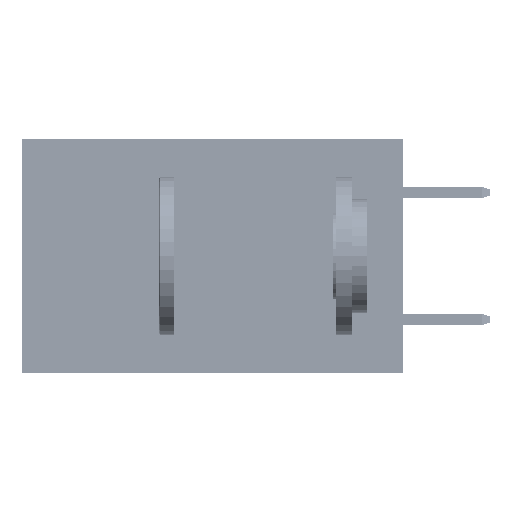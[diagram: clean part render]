
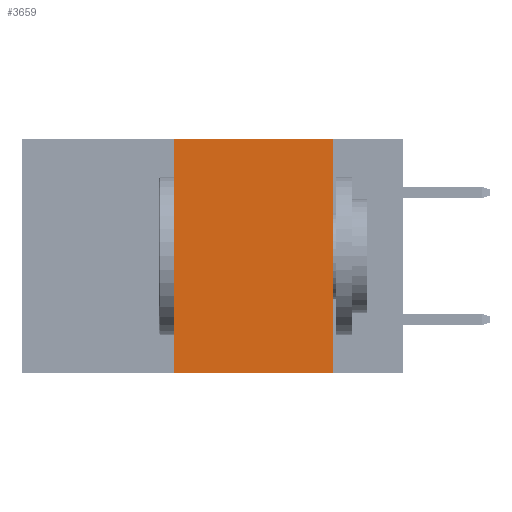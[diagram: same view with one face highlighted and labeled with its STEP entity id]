
A CAD part, left-side view. The second image highlights one B-rep face of the part: STEP entity #3659.
In plain terms, the highlighted planar face has unit normal (-1, 0, 0).
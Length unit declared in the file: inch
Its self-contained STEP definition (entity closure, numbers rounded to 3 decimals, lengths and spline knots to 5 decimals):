
#882 = EDGE_CURVE ( 'NONE', #18003, #34850, #11308, .T. ) ;
#1052 = DIRECTION ( 'NONE',  ( 0., -1., 0. ) ) ;
#3436 = DIRECTION ( 'NONE',  ( 0., -1., 0. ) ) ;
#3535 = DIRECTION ( 'NONE',  ( 0., 0., 1. ) ) ;
#3659 = ADVANCED_FACE ( 'NONE', ( #10987 ), #38958, .F. ) ;
#3893 = VERTEX_POINT ( 'NONE', #39725 ) ;
#4242 = LINE ( 'NONE', #36251, #7259 ) ;
#6133 = DIRECTION ( 'NONE',  ( 0., 0., -1. ) ) ;
#7259 = VECTOR ( 'NONE', #3436, 39.37008 ) ;
#8199 = CARTESIAN_POINT ( 'NONE',  ( 0., 0.36, 0. ) ) ;
#9303 = ORIENTED_EDGE ( 'NONE', *, *, #16327, .F. ) ;
#10695 = CARTESIAN_POINT ( 'NONE',  ( 0., 0.11, 0. ) ) ;
#10987 = FACE_OUTER_BOUND ( 'NONE', #26931, .T. ) ;
#11308 = LINE ( 'NONE', #41308, #29455 ) ;
#11446 = VECTOR ( 'NONE', #1052, 39.37008 ) ;
#14452 = DIRECTION ( 'NONE',  ( 1., 0., 0. ) ) ;
#16327 = EDGE_CURVE ( 'NONE', #3893, #21824, #34948, .T. ) ;
#18003 = VERTEX_POINT ( 'NONE', #46081 ) ;
#18189 = CARTESIAN_POINT ( 'NONE',  ( 0., 0.6, 0. ) ) ;
#19216 = DIRECTION ( 'NONE',  ( 0., 0., -1. ) ) ;
#21824 = VERTEX_POINT ( 'NONE', #35197 ) ;
#25587 = CARTESIAN_POINT ( 'NONE',  ( 0., 0.6, -0.37 ) ) ;
#26931 = EDGE_LOOP ( 'NONE', ( #9303, #37479, #32666, #40586 ) ) ;
#29455 = VECTOR ( 'NONE', #3535, 39.37008 ) ;
#29867 = LINE ( 'NONE', #25587, #11446 ) ;
#29952 = EDGE_CURVE ( 'NONE', #34850, #3893, #4242, .T. ) ;
#30561 = AXIS2_PLACEMENT_3D ( 'NONE', #18189, #14452, #19216 ) ;
#32666 = ORIENTED_EDGE ( 'NONE', *, *, #882, .F. ) ;
#34850 = VERTEX_POINT ( 'NONE', #8199 ) ;
#34948 = LINE ( 'NONE', #10695, #43179 ) ;
#35197 = CARTESIAN_POINT ( 'NONE',  ( 0., 0.11, -0.37 ) ) ;
#36251 = CARTESIAN_POINT ( 'NONE',  ( 0., 0.6, 0. ) ) ;
#37479 = ORIENTED_EDGE ( 'NONE', *, *, #29952, .F. ) ;
#38958 = PLANE ( 'NONE',  #30561 ) ;
#39236 = EDGE_CURVE ( 'NONE', #18003, #21824, #29867, .T. ) ;
#39725 = CARTESIAN_POINT ( 'NONE',  ( 0., 0.11, 0. ) ) ;
#40586 = ORIENTED_EDGE ( 'NONE', *, *, #39236, .T. ) ;
#41308 = CARTESIAN_POINT ( 'NONE',  ( 0., 0.36, 0. ) ) ;
#43179 = VECTOR ( 'NONE', #6133, 39.37008 ) ;
#46081 = CARTESIAN_POINT ( 'NONE',  ( 0., 0.36, -0.37 ) ) ;
